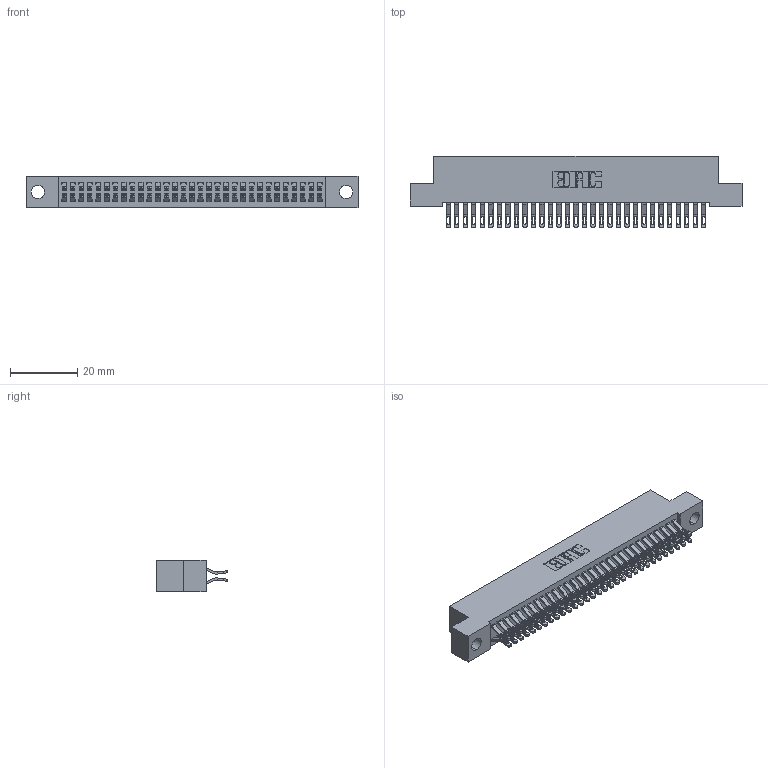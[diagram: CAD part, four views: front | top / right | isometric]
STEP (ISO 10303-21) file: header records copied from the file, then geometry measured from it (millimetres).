
FILE_DESCRIPTION (( 'STEP AP203' ), '1' );
FILE_NAME ('392-062-555-204.STEP', '2018-08-17T21:14:58', ( '' ), ( '' ), 'SwSTEP 2.0', 'SolidWorks 2016', '' );
FILE_SCHEMA (( 'CONFIG_CONTROL_DESIGN' ));
Length unit declared in the file: inch
Products named in the file (3): 342 Part_.156 TH; 345-292-001_555 Tail; 392-062-555-204
Assembly tree (63 placements, depth 2):
  392-062-555-204
    342 Part_.156 TH
    345-292-001_555 Tail  x62
Bounding box: 99.06 x 21.47 x 9.4 mm (x, y, z)
Volume: 8933.7 mm3; surface area: 14694.9 mm2
Topology: 63 solids, 63 shells, 3706 faces, 11645 edges, 7762 vertices
Faces by surface type: plane 2174, cylinder 1532
Entity records: 21563 total; most frequent: CARTESIAN_POINT 3620, ORIENTED_EDGE 3526, DIRECTION 3083, EDGE_CURVE 1763, LINE 1615, VECTOR 1615, VERTEX_POINT 1174, AXIS2_PLACEMENT_3D 734
